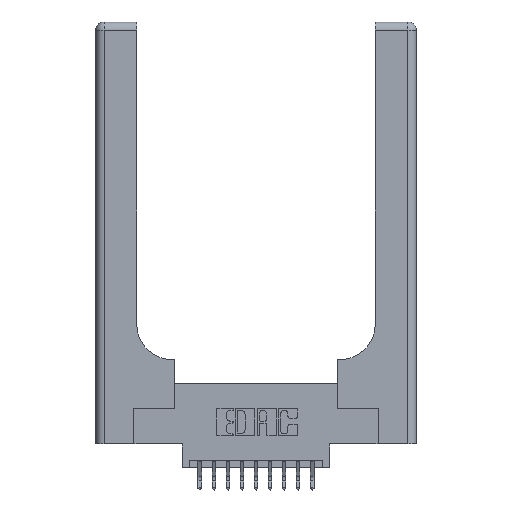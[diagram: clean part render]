
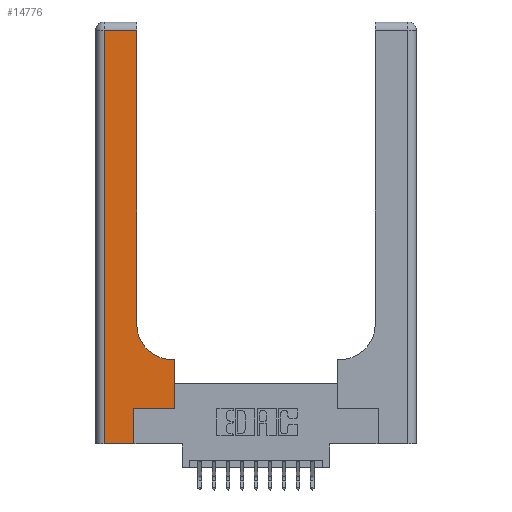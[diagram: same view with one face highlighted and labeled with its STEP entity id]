
A CAD part, top view. The second image highlights one B-rep face of the part: STEP entity #14776.
In plain terms, the highlighted planar face has unit normal (0, 0, 1).
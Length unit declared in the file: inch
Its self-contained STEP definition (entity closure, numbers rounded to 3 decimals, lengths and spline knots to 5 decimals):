
#88 = FACE_OUTER_BOUND ( 'NONE', #6459, .T. ) ;
#204 = LINE ( 'NONE', #2338, #10491 ) ;
#518 = VERTEX_POINT ( 'NONE', #6581 ) ;
#771 = ORIENTED_EDGE ( 'NONE', *, *, #12903, .T. ) ;
#883 = LINE ( 'NONE', #14981, #11110 ) ;
#952 = CARTESIAN_POINT ( 'NONE',  ( 0.5585, 0.6, 0.37 ) ) ;
#1204 = LINE ( 'NONE', #16852, #11014 ) ;
#1305 = LINE ( 'NONE', #6338, #5326 ) ;
#1319 = EDGE_CURVE ( 'NONE', #9131, #15638, #883, .T. ) ;
#1850 = VERTEX_POINT ( 'NONE', #9331 ) ;
#1928 = ORIENTED_EDGE ( 'NONE', *, *, #2091, .T. ) ;
#2091 = EDGE_CURVE ( 'NONE', #3068, #518, #1305, .T. ) ;
#2338 = CARTESIAN_POINT ( 'NONE',  ( 0.269, 0., 0.37 ) ) ;
#2357 = EDGE_CURVE ( 'NONE', #5368, #13771, #204, .T. ) ;
#2379 = DIRECTION ( 'NONE',  ( 1., 0., 0. ) ) ;
#2391 = DIRECTION ( 'NONE',  ( 0., 1., 0. ) ) ;
#2837 = CARTESIAN_POINT ( 'NONE',  ( 0.2915, 0.85, 0.37 ) ) ;
#3068 = VERTEX_POINT ( 'NONE', #952 ) ;
#3069 = VECTOR ( 'NONE', #2379, 39.37008 ) ;
#3336 = CARTESIAN_POINT ( 'NONE',  ( 0.06, 2.94, 0.37 ) ) ;
#3539 = LINE ( 'NONE', #13573, #14871 ) ;
#4119 = DIRECTION ( 'NONE',  ( 0., 0., -1. ) ) ;
#4276 = ORIENTED_EDGE ( 'NONE', *, *, #4761, .T. ) ;
#4363 = VECTOR ( 'NONE', #6771, 39.37008 ) ;
#4761 = EDGE_CURVE ( 'NONE', #518, #9131, #5029, .T. ) ;
#5029 = CIRCLE ( 'NONE', #13628, 0.25 ) ;
#5057 = EDGE_CURVE ( 'NONE', #7458, #5368, #1204, .T. ) ;
#5326 = VECTOR ( 'NONE', #6281, 39.37008 ) ;
#5368 = VERTEX_POINT ( 'NONE', #9800 ) ;
#6281 = DIRECTION ( 'NONE',  ( -1., 0., 0. ) ) ;
#6338 = CARTESIAN_POINT ( 'NONE',  ( 0.2915, 0.6, 0.37 ) ) ;
#6459 = EDGE_LOOP ( 'NONE', ( #6479, #12252, #771, #6530, #11266, #9662, #13848, #1928, #4276 ) ) ;
#6479 = ORIENTED_EDGE ( 'NONE', *, *, #1319, .T. ) ;
#6530 = ORIENTED_EDGE ( 'NONE', *, *, #5057, .T. ) ;
#6581 = CARTESIAN_POINT ( 'NONE',  ( 0.5415, 0.6, 0.37 ) ) ;
#6701 = DIRECTION ( 'NONE',  ( -1., 0., 0. ) ) ;
#6771 = DIRECTION ( 'NONE',  ( 0., -1., 0. ) ) ;
#6791 = LINE ( 'NONE', #9138, #3069 ) ;
#7378 = DIRECTION ( 'NONE',  ( 0., 0., -1. ) ) ;
#7458 = VERTEX_POINT ( 'NONE', #11196 ) ;
#7794 = EDGE_CURVE ( 'NONE', #15638, #15482, #10561, .T. ) ;
#7944 = CARTESIAN_POINT ( 'NONE',  ( 0., 2.94, 0.37 ) ) ;
#8120 = PLANE ( 'NONE',  #15988 ) ;
#8176 = CARTESIAN_POINT ( 'NONE',  ( 0., 3., 0.37 ) ) ;
#9131 = VERTEX_POINT ( 'NONE', #2837 ) ;
#9138 = CARTESIAN_POINT ( 'NONE',  ( 0.269, 0.25, 0.37 ) ) ;
#9331 = CARTESIAN_POINT ( 'NONE',  ( 0.5585, 0.25, 0.37 ) ) ;
#9662 = ORIENTED_EDGE ( 'NONE', *, *, #12057, .T. ) ;
#9800 = CARTESIAN_POINT ( 'NONE',  ( 0.269, 0., 0.37 ) ) ;
#9915 = EDGE_CURVE ( 'NONE', #1850, #3068, #3539, .T. ) ;
#10491 = VECTOR ( 'NONE', #2391, 39.37008 ) ;
#10561 = LINE ( 'NONE', #7944, #13581 ) ;
#11014 = VECTOR ( 'NONE', #11765, 39.37008 ) ;
#11040 = DIRECTION ( 'NONE',  ( 0., 1., 0. ) ) ;
#11110 = VECTOR ( 'NONE', #14976, 39.37008 ) ;
#11196 = CARTESIAN_POINT ( 'NONE',  ( 0.06, 0., 0.37 ) ) ;
#11266 = ORIENTED_EDGE ( 'NONE', *, *, #2357, .T. ) ;
#11765 = DIRECTION ( 'NONE',  ( 1., 0., 0. ) ) ;
#12057 = EDGE_CURVE ( 'NONE', #13771, #1850, #6791, .T. ) ;
#12252 = ORIENTED_EDGE ( 'NONE', *, *, #7794, .T. ) ;
#12903 = EDGE_CURVE ( 'NONE', #15482, #7458, #14831, .T. ) ;
#13370 = DIRECTION ( 'NONE',  ( -1., 0., 0. ) ) ;
#13573 = CARTESIAN_POINT ( 'NONE',  ( 0.5585, 0.25, 0.37 ) ) ;
#13581 = VECTOR ( 'NONE', #6701, 39.37008 ) ;
#13628 = AXIS2_PLACEMENT_3D ( 'NONE', #15088, #7378, #16368 ) ;
#13771 = VERTEX_POINT ( 'NONE', #16412 ) ;
#13841 = CARTESIAN_POINT ( 'NONE',  ( 0.2915, 2.94, 0.37 ) ) ;
#13848 = ORIENTED_EDGE ( 'NONE', *, *, #9915, .T. ) ;
#14776 = ADVANCED_FACE ( 'NONE', ( #88 ), #8120, .F. ) ;
#14831 = LINE ( 'NONE', #15774, #4363 ) ;
#14871 = VECTOR ( 'NONE', #11040, 39.37008 ) ;
#14976 = DIRECTION ( 'NONE',  ( 0., 1., 0. ) ) ;
#14981 = CARTESIAN_POINT ( 'NONE',  ( 0.2915, 3., 0.37 ) ) ;
#15088 = CARTESIAN_POINT ( 'NONE',  ( 0.5415, 0.85, 0.37 ) ) ;
#15482 = VERTEX_POINT ( 'NONE', #3336 ) ;
#15638 = VERTEX_POINT ( 'NONE', #13841 ) ;
#15774 = CARTESIAN_POINT ( 'NONE',  ( 0.06, 3., 0.37 ) ) ;
#15988 = AXIS2_PLACEMENT_3D ( 'NONE', #8176, #4119, #13370 ) ;
#16368 = DIRECTION ( 'NONE',  ( 1., 0., 0. ) ) ;
#16412 = CARTESIAN_POINT ( 'NONE',  ( 0.269, 0.25, 0.37 ) ) ;
#16852 = CARTESIAN_POINT ( 'NONE',  ( 0., 0., 0.37 ) ) ;
